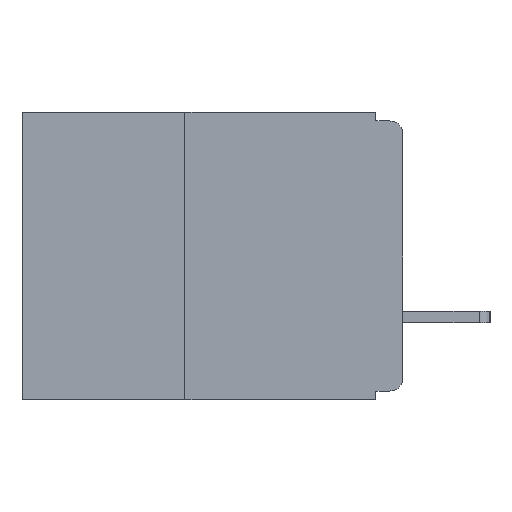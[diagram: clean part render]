
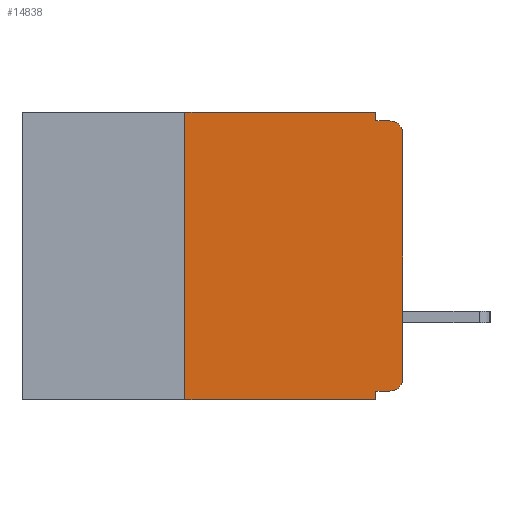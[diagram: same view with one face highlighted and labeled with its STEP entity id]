
A CAD part, left-side view. The second image highlights one B-rep face of the part: STEP entity #14838.
In plain terms, the highlighted planar face has unit normal (-1, 0, 0).
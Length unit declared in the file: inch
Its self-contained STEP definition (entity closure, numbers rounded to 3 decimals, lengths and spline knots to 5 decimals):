
#329 = EDGE_CURVE ( 'NONE', #12839, #649, #13068, .T. ) ;
#649 = VERTEX_POINT ( 'NONE', #24634 ) ;
#750 = CARTESIAN_POINT ( 'NONE',  ( 0., 0., -0.01 ) ) ;
#828 = ORIENTED_EDGE ( 'NONE', *, *, #10995, .F. ) ;
#829 = EDGE_CURVE ( 'NONE', #12839, #18435, #21450, .T. ) ;
#1277 = PLANE ( 'NONE',  #1360 ) ;
#1360 = AXIS2_PLACEMENT_3D ( 'NONE', #3251, #5192, #18541 ) ;
#1574 = VECTOR ( 'NONE', #24521, 39.37008 ) ;
#2496 = VECTOR ( 'NONE', #23291, 39.37008 ) ;
#2783 = DIRECTION ( 'NONE',  ( -1., 0., 0. ) ) ;
#2815 = EDGE_CURVE ( 'NONE', #6202, #4612, #3104, .T. ) ;
#2875 = DIRECTION ( 'NONE',  ( 0., 0., -1. ) ) ;
#3104 = LINE ( 'NONE', #23770, #2496 ) ;
#3251 = CARTESIAN_POINT ( 'NONE',  ( 0., 0.437, 0. ) ) ;
#3266 = CARTESIAN_POINT ( 'NONE',  ( 0., 0.437, -0.33 ) ) ;
#3808 = EDGE_CURVE ( 'NONE', #649, #14914, #14443, .T. ) ;
#4035 = ORIENTED_EDGE ( 'NONE', *, *, #7541, .F. ) ;
#4157 = ORIENTED_EDGE ( 'NONE', *, *, #21209, .F. ) ;
#4252 = CARTESIAN_POINT ( 'NONE',  ( 0., 0.015, -0.01 ) ) ;
#4327 = CARTESIAN_POINT ( 'NONE',  ( 0., 0., -0.32 ) ) ;
#4612 = VERTEX_POINT ( 'NONE', #9688 ) ;
#4852 = CARTESIAN_POINT ( 'NONE',  ( 0., 0.015, -0.305 ) ) ;
#4907 = VECTOR ( 'NONE', #14697, 39.37008 ) ;
#5192 = DIRECTION ( 'NONE',  ( 1., 0., 0. ) ) ;
#5416 = ORIENTED_EDGE ( 'NONE', *, *, #8939, .F. ) ;
#6202 = VERTEX_POINT ( 'NONE', #15314 ) ;
#6603 = DIRECTION ( 'NONE',  ( 0., -1., 0. ) ) ;
#6789 = DIRECTION ( 'NONE',  ( 0., 0., -1. ) ) ;
#6818 = DIRECTION ( 'NONE',  ( 0., -1., 0. ) ) ;
#6835 = VECTOR ( 'NONE', #6818, 39.37008 ) ;
#7473 = CARTESIAN_POINT ( 'NONE',  ( 0., 0.031, -0.33 ) ) ;
#7541 = EDGE_CURVE ( 'NONE', #10563, #21584, #24399, .T. ) ;
#8062 = VECTOR ( 'NONE', #15645, 39.37008 ) ;
#8939 = EDGE_CURVE ( 'NONE', #14842, #18435, #16256, .T. ) ;
#9074 = AXIS2_PLACEMENT_3D ( 'NONE', #4852, #18185, #6789 ) ;
#9688 = CARTESIAN_POINT ( 'NONE',  ( 0., 0., -0.025 ) ) ;
#9709 = ORIENTED_EDGE ( 'NONE', *, *, #2815, .T. ) ;
#10563 = VERTEX_POINT ( 'NONE', #16348 ) ;
#10809 = EDGE_LOOP ( 'NONE', ( #9709, #10895, #4035, #4157, #12730, #19379, #17040, #5416, #828, #18660 ) ) ;
#10895 = ORIENTED_EDGE ( 'NONE', *, *, #21167, .T. ) ;
#10995 = EDGE_CURVE ( 'NONE', #13557, #14842, #12189, .T. ) ;
#11947 = VECTOR ( 'NONE', #15736, 39.37008 ) ;
#12158 = CIRCLE ( 'NONE', #9074, 0.015 ) ;
#12189 = LINE ( 'NONE', #4327, #11947 ) ;
#12363 = CARTESIAN_POINT ( 'NONE',  ( 0., 0.031, 0. ) ) ;
#12730 = ORIENTED_EDGE ( 'NONE', *, *, #3808, .F. ) ;
#12741 = CARTESIAN_POINT ( 'NONE',  ( 0., 0.031, -0.32 ) ) ;
#12839 = VERTEX_POINT ( 'NONE', #23981 ) ;
#12999 = CARTESIAN_POINT ( 'NONE',  ( 0., 0.437, 0. ) ) ;
#13068 = LINE ( 'NONE', #14021, #8062 ) ;
#13557 = VERTEX_POINT ( 'NONE', #20370 ) ;
#14021 = CARTESIAN_POINT ( 'NONE',  ( 0., 0.25, -0.33 ) ) ;
#14236 = CARTESIAN_POINT ( 'NONE',  ( 0., 0.015, -0.025 ) ) ;
#14443 = LINE ( 'NONE', #12999, #4907 ) ;
#14697 = DIRECTION ( 'NONE',  ( 0., -1., 0. ) ) ;
#14825 = VECTOR ( 'NONE', #2875, 39.37008 ) ;
#14838 = ADVANCED_FACE ( 'NONE', ( #16217 ), #1277, .F. ) ;
#14842 = VERTEX_POINT ( 'NONE', #12741 ) ;
#14914 = VERTEX_POINT ( 'NONE', #24431 ) ;
#15314 = CARTESIAN_POINT ( 'NONE',  ( 0., 0., -0.305 ) ) ;
#15645 = DIRECTION ( 'NONE',  ( 0., 0., 1. ) ) ;
#15735 = AXIS2_PLACEMENT_3D ( 'NONE', #14236, #2783, #16140 ) ;
#15736 = DIRECTION ( 'NONE',  ( 0., 1., 0. ) ) ;
#16140 = DIRECTION ( 'NONE',  ( 0., 0., -1. ) ) ;
#16217 = FACE_OUTER_BOUND ( 'NONE', #10809, .T. ) ;
#16256 = LINE ( 'NONE', #24453, #1574 ) ;
#16348 = CARTESIAN_POINT ( 'NONE',  ( 0., 0.031, -0.01 ) ) ;
#17040 = ORIENTED_EDGE ( 'NONE', *, *, #829, .T. ) ;
#18185 = DIRECTION ( 'NONE',  ( -1., 0., 0. ) ) ;
#18435 = VERTEX_POINT ( 'NONE', #7473 ) ;
#18541 = DIRECTION ( 'NONE',  ( 0., 0., -1. ) ) ;
#18660 = ORIENTED_EDGE ( 'NONE', *, *, #20586, .T. ) ;
#19379 = ORIENTED_EDGE ( 'NONE', *, *, #329, .F. ) ;
#19950 = LINE ( 'NONE', #12363, #14825 ) ;
#20370 = CARTESIAN_POINT ( 'NONE',  ( 0., 0.015, -0.32 ) ) ;
#20586 = EDGE_CURVE ( 'NONE', #13557, #6202, #12158, .T. ) ;
#21142 = CIRCLE ( 'NONE', #15735, 0.015 ) ;
#21167 = EDGE_CURVE ( 'NONE', #4612, #21584, #21142, .T. ) ;
#21209 = EDGE_CURVE ( 'NONE', #14914, #10563, #19950, .T. ) ;
#21450 = LINE ( 'NONE', #3266, #6835 ) ;
#21584 = VERTEX_POINT ( 'NONE', #4252 ) ;
#23291 = DIRECTION ( 'NONE',  ( 0., 0., 1. ) ) ;
#23770 = CARTESIAN_POINT ( 'NONE',  ( 0., 0., 0. ) ) ;
#23831 = VECTOR ( 'NONE', #6603, 39.37008 ) ;
#23981 = CARTESIAN_POINT ( 'NONE',  ( 0., 0.25, -0.33 ) ) ;
#24399 = LINE ( 'NONE', #750, #23831 ) ;
#24431 = CARTESIAN_POINT ( 'NONE',  ( 0., 0.031, 0. ) ) ;
#24453 = CARTESIAN_POINT ( 'NONE',  ( 0., 0.031, -0.33 ) ) ;
#24521 = DIRECTION ( 'NONE',  ( 0., 0., -1. ) ) ;
#24634 = CARTESIAN_POINT ( 'NONE',  ( 0., 0.25, 0. ) ) ;
